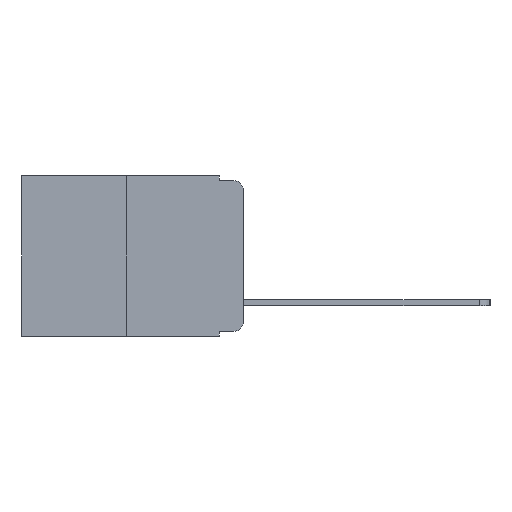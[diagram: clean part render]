
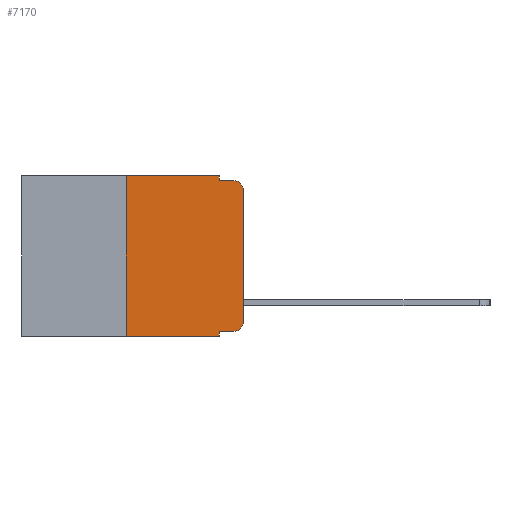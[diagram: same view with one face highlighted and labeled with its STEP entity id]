
A CAD part, left-side view. The second image highlights one B-rep face of the part: STEP entity #7170.
In plain terms, the highlighted planar face has unit normal (-1, 0, 0).
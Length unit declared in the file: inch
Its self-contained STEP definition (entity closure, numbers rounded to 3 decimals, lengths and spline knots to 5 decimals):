
#111 = VERTEX_POINT ( 'NONE', #17357 ) ;
#322 = VECTOR ( 'NONE', #11315, 39.37008 ) ;
#342 = ORIENTED_EDGE ( 'NONE', *, *, #7190, .T. ) ;
#348 = EDGE_CURVE ( 'NONE', #17936, #1866, #893, .T. ) ;
#588 = ORIENTED_EDGE ( 'NONE', *, *, #18361, .T. ) ;
#893 = LINE ( 'NONE', #18162, #15710 ) ;
#1134 = ORIENTED_EDGE ( 'NONE', *, *, #5804, .F. ) ;
#1135 = DIRECTION ( 'NONE',  ( 0., 0., -1. ) ) ;
#1240 = CARTESIAN_POINT ( 'NONE',  ( 0., 0.25, 0. ) ) ;
#1251 = VECTOR ( 'NONE', #4240, 39.37008 ) ;
#1866 = VERTEX_POINT ( 'NONE', #4471 ) ;
#2069 = CARTESIAN_POINT ( 'NONE',  ( 0., 0.02, -0.313 ) ) ;
#2083 = CARTESIAN_POINT ( 'NONE',  ( 0., 0., -0.03 ) ) ;
#2226 = VERTEX_POINT ( 'NONE', #15261 ) ;
#2376 = CARTESIAN_POINT ( 'NONE',  ( 0., 0.051, -0.01 ) ) ;
#2429 = EDGE_CURVE ( 'NONE', #17846, #12116, #14100, .T. ) ;
#2514 = DIRECTION ( 'NONE',  ( 0., -1., 0. ) ) ;
#2742 = LINE ( 'NONE', #4049, #10477 ) ;
#2971 = DIRECTION ( 'NONE',  ( 0., 0., -1. ) ) ;
#3079 = EDGE_CURVE ( 'NONE', #13448, #17846, #11474, .T. ) ;
#3677 = DIRECTION ( 'NONE',  ( 0., 0., -1. ) ) ;
#4049 = CARTESIAN_POINT ( 'NONE',  ( 0., 0.25, 0. ) ) ;
#4240 = DIRECTION ( 'NONE',  ( 0., 0., 1. ) ) ;
#4268 = LINE ( 'NONE', #15453, #322 ) ;
#4471 = CARTESIAN_POINT ( 'NONE',  ( 0., 0.051, -0.343 ) ) ;
#4912 = ORIENTED_EDGE ( 'NONE', *, *, #348, .T. ) ;
#5582 = DIRECTION ( 'NONE',  ( 0., -1., 0. ) ) ;
#5804 = EDGE_CURVE ( 'NONE', #17936, #13448, #2742, .T. ) ;
#6116 = CARTESIAN_POINT ( 'NONE',  ( 0., 0.051, 0. ) ) ;
#6165 = DIRECTION ( 'NONE',  ( -1., 0., 0. ) ) ;
#6431 = ORIENTED_EDGE ( 'NONE', *, *, #2429, .F. ) ;
#6483 = VECTOR ( 'NONE', #16604, 39.37008 ) ;
#6706 = CARTESIAN_POINT ( 'NONE',  ( 0., 0.051, -0.333 ) ) ;
#7170 = ADVANCED_FACE ( 'NONE', ( #16951 ), #8442, .F. ) ;
#7190 = EDGE_CURVE ( 'NONE', #12050, #2226, #13273, .T. ) ;
#7700 = VECTOR ( 'NONE', #15529, 39.37008 ) ;
#8391 = CARTESIAN_POINT ( 'NONE',  ( 0., 0.02, -0.01 ) ) ;
#8442 = PLANE ( 'NONE',  #11711 ) ;
#9632 = ORIENTED_EDGE ( 'NONE', *, *, #13459, .T. ) ;
#9905 = DIRECTION ( 'NONE',  ( 1., 0., 0. ) ) ;
#10344 = ORIENTED_EDGE ( 'NONE', *, *, #11339, .T. ) ;
#10477 = VECTOR ( 'NONE', #14019, 39.37008 ) ;
#10841 = VECTOR ( 'NONE', #2971, 39.37008 ) ;
#10905 = VERTEX_POINT ( 'NONE', #2083 ) ;
#11245 = CARTESIAN_POINT ( 'NONE',  ( 0., 0.051, -0.333 ) ) ;
#11315 = DIRECTION ( 'NONE',  ( 0., 0., -1. ) ) ;
#11339 = EDGE_CURVE ( 'NONE', #2226, #111, #18567, .T. ) ;
#11474 = LINE ( 'NONE', #18294, #7700 ) ;
#11618 = CARTESIAN_POINT ( 'NONE',  ( 0., 0.051, 0. ) ) ;
#11711 = AXIS2_PLACEMENT_3D ( 'NONE', #14035, #9905, #1135 ) ;
#11981 = CARTESIAN_POINT ( 'NONE',  ( 0., 0.25, -0.343 ) ) ;
#12050 = VERTEX_POINT ( 'NONE', #6706 ) ;
#12101 = AXIS2_PLACEMENT_3D ( 'NONE', #2069, #12165, #3677 ) ;
#12116 = VERTEX_POINT ( 'NONE', #16741 ) ;
#12165 = DIRECTION ( 'NONE',  ( -1., 0., 0. ) ) ;
#12779 = LINE ( 'NONE', #14201, #1251 ) ;
#13019 = AXIS2_PLACEMENT_3D ( 'NONE', #14668, #6165, #16069 ) ;
#13273 = LINE ( 'NONE', #11245, #16529 ) ;
#13448 = VERTEX_POINT ( 'NONE', #1240 ) ;
#13459 = EDGE_CURVE ( 'NONE', #111, #10905, #12779, .T. ) ;
#13781 = CIRCLE ( 'NONE', #13019, 0.02 ) ;
#14019 = DIRECTION ( 'NONE',  ( 0., 0., 1. ) ) ;
#14035 = CARTESIAN_POINT ( 'NONE',  ( 0., 0.473, 0. ) ) ;
#14100 = LINE ( 'NONE', #11618, #10841 ) ;
#14201 = CARTESIAN_POINT ( 'NONE',  ( 0., 0., 0. ) ) ;
#14296 = EDGE_LOOP ( 'NONE', ( #9632, #588, #16406, #6431, #17020, #1134, #4912, #15040, #342, #10344 ) ) ;
#14668 = CARTESIAN_POINT ( 'NONE',  ( 0., 0.02, -0.03 ) ) ;
#14859 = VERTEX_POINT ( 'NONE', #8391 ) ;
#15040 = ORIENTED_EDGE ( 'NONE', *, *, #16576, .F. ) ;
#15261 = CARTESIAN_POINT ( 'NONE',  ( 0., 0.02, -0.333 ) ) ;
#15453 = CARTESIAN_POINT ( 'NONE',  ( 0., 0.051, 0. ) ) ;
#15529 = DIRECTION ( 'NONE',  ( 0., -1., 0. ) ) ;
#15710 = VECTOR ( 'NONE', #2514, 39.37008 ) ;
#16069 = DIRECTION ( 'NONE',  ( 0., 0., -1. ) ) ;
#16406 = ORIENTED_EDGE ( 'NONE', *, *, #18116, .F. ) ;
#16529 = VECTOR ( 'NONE', #5582, 39.37008 ) ;
#16576 = EDGE_CURVE ( 'NONE', #12050, #1866, #4268, .T. ) ;
#16604 = DIRECTION ( 'NONE',  ( 0., -1., 0. ) ) ;
#16741 = CARTESIAN_POINT ( 'NONE',  ( 0., 0.051, -0.01 ) ) ;
#16951 = FACE_OUTER_BOUND ( 'NONE', #14296, .T. ) ;
#17020 = ORIENTED_EDGE ( 'NONE', *, *, #3079, .F. ) ;
#17357 = CARTESIAN_POINT ( 'NONE',  ( 0., 0., -0.313 ) ) ;
#17732 = LINE ( 'NONE', #2376, #6483 ) ;
#17846 = VERTEX_POINT ( 'NONE', #6116 ) ;
#17936 = VERTEX_POINT ( 'NONE', #11981 ) ;
#18116 = EDGE_CURVE ( 'NONE', #12116, #14859, #17732, .T. ) ;
#18162 = CARTESIAN_POINT ( 'NONE',  ( 0., 0.473, -0.343 ) ) ;
#18294 = CARTESIAN_POINT ( 'NONE',  ( 0., 0.473, 0. ) ) ;
#18361 = EDGE_CURVE ( 'NONE', #10905, #14859, #13781, .T. ) ;
#18567 = CIRCLE ( 'NONE', #12101, 0.02 ) ;
